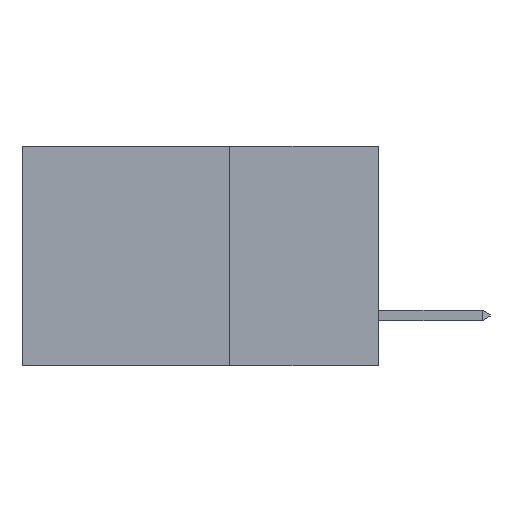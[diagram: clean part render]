
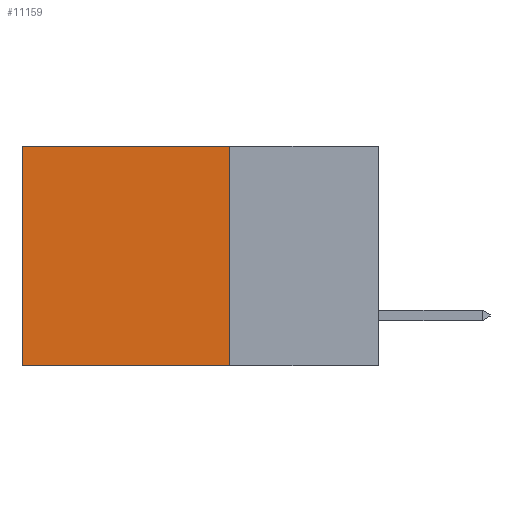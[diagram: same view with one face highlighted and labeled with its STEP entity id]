
A CAD part, left-side view. The second image highlights one B-rep face of the part: STEP entity #11159.
In plain terms, the highlighted planar face has unit normal (-1, 0, 0).
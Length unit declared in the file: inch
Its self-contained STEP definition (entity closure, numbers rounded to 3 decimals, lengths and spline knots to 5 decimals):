
#1670 = EDGE_CURVE ( 'NONE', #15093, #17310, #15458, .T. ) ;
#1923 = EDGE_LOOP ( 'NONE', ( #2290, #10269, #17836, #4089 ) ) ;
#2089 = CARTESIAN_POINT ( 'NONE',  ( 0.2615, 0.25, 0. ) ) ;
#2290 = ORIENTED_EDGE ( 'NONE', *, *, #5019, .T. ) ;
#3260 = CARTESIAN_POINT ( 'NONE',  ( 0.2615, 0.6, -0.37 ) ) ;
#3762 = VECTOR ( 'NONE', #19433, 39.37008 ) ;
#3972 = EDGE_CURVE ( 'NONE', #15093, #5789, #8625, .T. ) ;
#4089 = ORIENTED_EDGE ( 'NONE', *, *, #3972, .T. ) ;
#4691 = AXIS2_PLACEMENT_3D ( 'NONE', #10916, #10889, #10864 ) ;
#5019 = EDGE_CURVE ( 'NONE', #5789, #13016, #22354, .T. ) ;
#5079 = VECTOR ( 'NONE', #11091, 39.37008 ) ;
#5084 = CARTESIAN_POINT ( 'NONE',  ( 0.2615, 0.25, -0.37 ) ) ;
#5789 = VERTEX_POINT ( 'NONE', #11829 ) ;
#8625 = LINE ( 'NONE', #20109, #3762 ) ;
#9130 = LINE ( 'NONE', #11979, #18323 ) ;
#10269 = ORIENTED_EDGE ( 'NONE', *, *, #22801, .F. ) ;
#10864 = DIRECTION ( 'NONE',  ( 0., 0., -1. ) ) ;
#10889 = DIRECTION ( 'NONE',  ( 1., 0., 0. ) ) ;
#10916 = CARTESIAN_POINT ( 'NONE',  ( 0.2615, 0.25, -0.37 ) ) ;
#11091 = DIRECTION ( 'NONE',  ( 0., 0., -1. ) ) ;
#11159 = ADVANCED_FACE ( 'NONE', ( #11765 ), #11171, .F. ) ;
#11171 = PLANE ( 'NONE',  #4691 ) ;
#11765 = FACE_OUTER_BOUND ( 'NONE', #1923, .T. ) ;
#11829 = CARTESIAN_POINT ( 'NONE',  ( 0.2615, 0.6, 0. ) ) ;
#11979 = CARTESIAN_POINT ( 'NONE',  ( 0.2615, 0.25, -0.37 ) ) ;
#12773 = DIRECTION ( 'NONE',  ( 0., 0., -1. ) ) ;
#13016 = VERTEX_POINT ( 'NONE', #3260 ) ;
#13799 = DIRECTION ( 'NONE',  ( 0., 1., 0. ) ) ;
#14299 = CARTESIAN_POINT ( 'NONE',  ( 0.2615, 0.6, -0.37 ) ) ;
#15093 = VERTEX_POINT ( 'NONE', #2089 ) ;
#15458 = LINE ( 'NONE', #15693, #5079 ) ;
#15693 = CARTESIAN_POINT ( 'NONE',  ( 0.2615, 0.25, -0.37 ) ) ;
#17310 = VERTEX_POINT ( 'NONE', #5084 ) ;
#17477 = VECTOR ( 'NONE', #12773, 39.37008 ) ;
#17836 = ORIENTED_EDGE ( 'NONE', *, *, #1670, .F. ) ;
#18323 = VECTOR ( 'NONE', #13799, 39.37008 ) ;
#19433 = DIRECTION ( 'NONE',  ( 0., 1., 0. ) ) ;
#20109 = CARTESIAN_POINT ( 'NONE',  ( 0.2615, 0.25, 0. ) ) ;
#22354 = LINE ( 'NONE', #14299, #17477 ) ;
#22801 = EDGE_CURVE ( 'NONE', #17310, #13016, #9130, .T. ) ;
